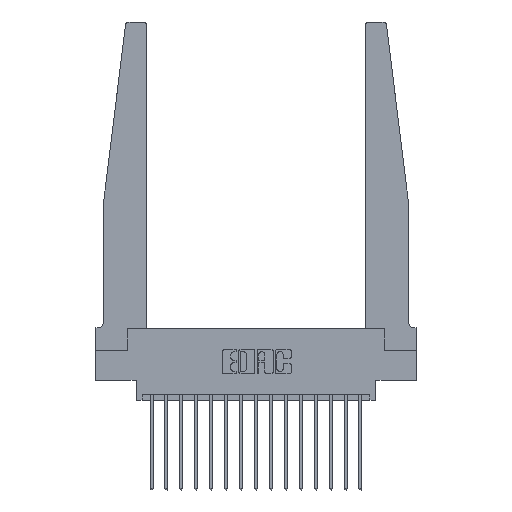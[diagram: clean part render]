
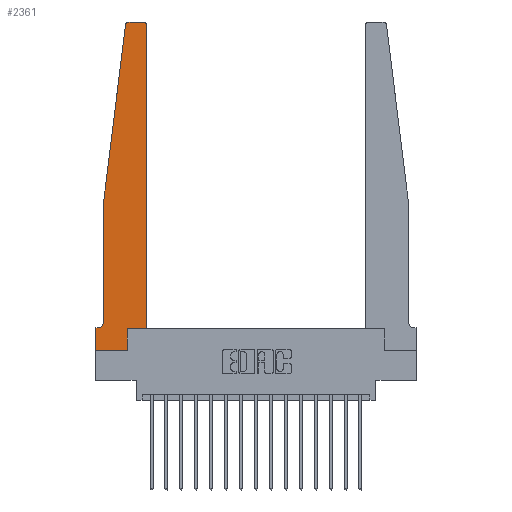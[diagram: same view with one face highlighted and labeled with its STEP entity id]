
A CAD part, top view. The second image highlights one B-rep face of the part: STEP entity #2361.
In plain terms, the highlighted planar face has unit normal (0, 0, 1).
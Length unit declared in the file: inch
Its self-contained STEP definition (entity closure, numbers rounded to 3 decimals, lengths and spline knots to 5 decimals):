
#20 = CARTESIAN_POINT ( 'NONE',  ( 0.425, 2.72, 0.37 ) ) ;
#50 = VECTOR ( 'NONE', #2394, 39.37008 ) ;
#248 = ORIENTED_EDGE ( 'NONE', *, *, #9042, .T. ) ;
#663 = PLANE ( 'NONE',  #10312 ) ;
#1032 = LINE ( 'NONE', #18699, #4333 ) ;
#1161 = VECTOR ( 'NONE', #10877, 39.37008 ) ;
#1289 = CARTESIAN_POINT ( 'NONE',  ( 0.065, 1.25, 0.37 ) ) ;
#1399 = VERTEX_POINT ( 'NONE', #5087 ) ;
#1854 = VERTEX_POINT ( 'NONE', #7659 ) ;
#1925 = EDGE_CURVE ( 'NONE', #15508, #1854, #11066, .T. ) ;
#2045 = ORIENTED_EDGE ( 'NONE', *, *, #1925, .T. ) ;
#2142 = AXIS2_PLACEMENT_3D ( 'NONE', #5438, #11240, #5521 ) ;
#2223 = CARTESIAN_POINT ( 'NONE',  ( 0.27653, 2.75, 0.37 ) ) ;
#2361 = ADVANCED_FACE ( 'NONE', ( #4953 ), #663, .T. ) ;
#2394 = DIRECTION ( 'NONE',  ( -1., 0., 0. ) ) ;
#2447 = EDGE_CURVE ( 'NONE', #1854, #3231, #6927, .T. ) ;
#2764 = CARTESIAN_POINT ( 'NONE',  ( 0., 0., 0.37 ) ) ;
#2788 = LINE ( 'NONE', #15805, #12205 ) ;
#3231 = VERTEX_POINT ( 'NONE', #12741 ) ;
#3362 = CARTESIAN_POINT ( 'NONE',  ( 0.015, 0.1875, 0.37 ) ) ;
#3481 = CARTESIAN_POINT ( 'NONE',  ( 0.065, 0.2375, 0.37 ) ) ;
#3669 = VERTEX_POINT ( 'NONE', #8619 ) ;
#3692 = VECTOR ( 'NONE', #5790, 39.37008 ) ;
#4086 = ORIENTED_EDGE ( 'NONE', *, *, #12736, .T. ) ;
#4123 = DIRECTION ( 'NONE',  ( -0.122, -0.992, 0. ) ) ;
#4207 = AXIS2_PLACEMENT_3D ( 'NONE', #6650, #6554, #5227 ) ;
#4333 = VECTOR ( 'NONE', #14427, 39.37008 ) ;
#4352 = LINE ( 'NONE', #8854, #11021 ) ;
#4953 = FACE_OUTER_BOUND ( 'NONE', #16711, .T. ) ;
#5046 = ORIENTED_EDGE ( 'NONE', *, *, #9878, .T. ) ;
#5087 = CARTESIAN_POINT ( 'NONE',  ( 0.065, 1.25, 0.37 ) ) ;
#5128 = VECTOR ( 'NONE', #7194, 39.37008 ) ;
#5227 = DIRECTION ( 'NONE',  ( -1., 0., 0. ) ) ;
#5245 = LINE ( 'NONE', #10962, #50 ) ;
#5438 = CARTESIAN_POINT ( 'NONE',  ( 0.27653, 2.72, 0.37 ) ) ;
#5506 = DIRECTION ( 'NONE',  ( 0., 1., 0. ) ) ;
#5521 = DIRECTION ( 'NONE',  ( 1., 0., 0. ) ) ;
#5790 = DIRECTION ( 'NONE',  ( 0., -1., 0. ) ) ;
#6032 = ORIENTED_EDGE ( 'NONE', *, *, #8519, .T. ) ;
#6231 = ORIENTED_EDGE ( 'NONE', *, *, #7140, .T. ) ;
#6554 = DIRECTION ( 'NONE',  ( 0., 0., -1. ) ) ;
#6650 = CARTESIAN_POINT ( 'NONE',  ( 0.015, 0.2375, 0.37 ) ) ;
#6927 = LINE ( 'NONE', #18420, #10635 ) ;
#7003 = LINE ( 'NONE', #1289, #15800 ) ;
#7107 = LINE ( 'NONE', #15552, #5128 ) ;
#7116 = VERTEX_POINT ( 'NONE', #20 ) ;
#7140 = EDGE_CURVE ( 'NONE', #7116, #3669, #15024, .T. ) ;
#7194 = DIRECTION ( 'NONE',  ( -1., 0., 0. ) ) ;
#7659 = CARTESIAN_POINT ( 'NONE',  ( 0.2605, 0., 0.37 ) ) ;
#7815 = ORIENTED_EDGE ( 'NONE', *, *, #14073, .T. ) ;
#8153 = VERTEX_POINT ( 'NONE', #18177 ) ;
#8394 = CARTESIAN_POINT ( 'NONE',  ( 0., 0., 0.37 ) ) ;
#8519 = EDGE_CURVE ( 'NONE', #3669, #15419, #5245, .T. ) ;
#8619 = CARTESIAN_POINT ( 'NONE',  ( 0.395, 2.75, 0.37 ) ) ;
#8742 = EDGE_CURVE ( 'NONE', #8153, #15508, #11502, .T. ) ;
#8854 = CARTESIAN_POINT ( 'NONE',  ( 0.425, 0.18, 0.37 ) ) ;
#9042 = EDGE_CURVE ( 'NONE', #3231, #17169, #4352, .T. ) ;
#9619 = CARTESIAN_POINT ( 'NONE',  ( 0.425, 0.18, 0.37 ) ) ;
#9878 = EDGE_CURVE ( 'NONE', #17169, #7116, #1032, .T. ) ;
#10312 = AXIS2_PLACEMENT_3D ( 'NONE', #12082, #12179, #13696 ) ;
#10560 = ORIENTED_EDGE ( 'NONE', *, *, #8742, .T. ) ;
#10635 = VECTOR ( 'NONE', #5506, 39.37008 ) ;
#10796 = AXIS2_PLACEMENT_3D ( 'NONE', #12957, #15697, #14282 ) ;
#10877 = DIRECTION ( 'NONE',  ( 1., 0., 0. ) ) ;
#10962 = CARTESIAN_POINT ( 'NONE',  ( 0.25, 2.75, 0.37 ) ) ;
#10971 = CARTESIAN_POINT ( 'NONE',  ( 0., 0., 0.37 ) ) ;
#11021 = VECTOR ( 'NONE', #14626, 39.37008 ) ;
#11066 = LINE ( 'NONE', #10971, #1161 ) ;
#11240 = DIRECTION ( 'NONE',  ( 0., 0., 1. ) ) ;
#11502 = LINE ( 'NONE', #8394, #3692 ) ;
#11761 = ORIENTED_EDGE ( 'NONE', *, *, #16271, .T. ) ;
#11860 = VERTEX_POINT ( 'NONE', #3481 ) ;
#12082 = CARTESIAN_POINT ( 'NONE',  ( 0., 0.1875, 0.37 ) ) ;
#12179 = DIRECTION ( 'NONE',  ( 0., 0., 1. ) ) ;
#12205 = VECTOR ( 'NONE', #17222, 39.37008 ) ;
#12736 = EDGE_CURVE ( 'NONE', #11860, #16459, #15157, .T. ) ;
#12741 = CARTESIAN_POINT ( 'NONE',  ( 0.2605, 0.18, 0.37 ) ) ;
#12957 = CARTESIAN_POINT ( 'NONE',  ( 0.395, 2.72, 0.37 ) ) ;
#13696 = DIRECTION ( 'NONE',  ( 1., 0., 0. ) ) ;
#13741 = ORIENTED_EDGE ( 'NONE', *, *, #14383, .T. ) ;
#13910 = VERTEX_POINT ( 'NONE', #16648 ) ;
#14073 = EDGE_CURVE ( 'NONE', #15419, #13910, #18514, .T. ) ;
#14282 = DIRECTION ( 'NONE',  ( 1., 0., 0. ) ) ;
#14383 = EDGE_CURVE ( 'NONE', #13910, #1399, #7003, .T. ) ;
#14427 = DIRECTION ( 'NONE',  ( 0., 1., 0. ) ) ;
#14626 = DIRECTION ( 'NONE',  ( 1., 0., 0. ) ) ;
#15024 = CIRCLE ( 'NONE', #10796, 0.03 ) ;
#15157 = CIRCLE ( 'NONE', #4207, 0.05 ) ;
#15419 = VERTEX_POINT ( 'NONE', #2223 ) ;
#15508 = VERTEX_POINT ( 'NONE', #2764 ) ;
#15552 = CARTESIAN_POINT ( 'NONE',  ( 0.065, 0.1875, 0.37 ) ) ;
#15697 = DIRECTION ( 'NONE',  ( 0., 0., 1. ) ) ;
#15800 = VECTOR ( 'NONE', #4123, 39.37008 ) ;
#15805 = CARTESIAN_POINT ( 'NONE',  ( 0.065, 1.25, 0.37 ) ) ;
#16271 = EDGE_CURVE ( 'NONE', #1399, #11860, #2788, .T. ) ;
#16459 = VERTEX_POINT ( 'NONE', #3362 ) ;
#16488 = ORIENTED_EDGE ( 'NONE', *, *, #18645, .T. ) ;
#16648 = CARTESIAN_POINT ( 'NONE',  ( 0.24675, 2.72367, 0.37 ) ) ;
#16711 = EDGE_LOOP ( 'NONE', ( #6032, #7815, #13741, #11761, #4086, #16488, #10560, #2045, #18573, #248, #5046, #6231 ) ) ;
#17169 = VERTEX_POINT ( 'NONE', #9619 ) ;
#17222 = DIRECTION ( 'NONE',  ( 0., -1., 0. ) ) ;
#18177 = CARTESIAN_POINT ( 'NONE',  ( 0., 0.1875, 0.37 ) ) ;
#18420 = CARTESIAN_POINT ( 'NONE',  ( 0.2605, 0.18, 0.37 ) ) ;
#18514 = CIRCLE ( 'NONE', #2142, 0.03 ) ;
#18573 = ORIENTED_EDGE ( 'NONE', *, *, #2447, .T. ) ;
#18645 = EDGE_CURVE ( 'NONE', #16459, #8153, #7107, .T. ) ;
#18699 = CARTESIAN_POINT ( 'NONE',  ( 0.425, 0.18, 0.37 ) ) ;
